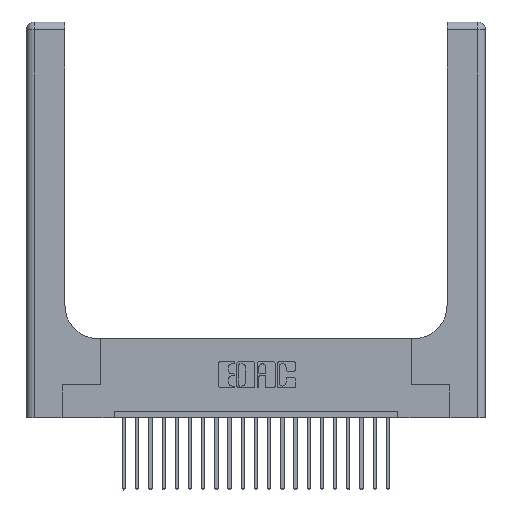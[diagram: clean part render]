
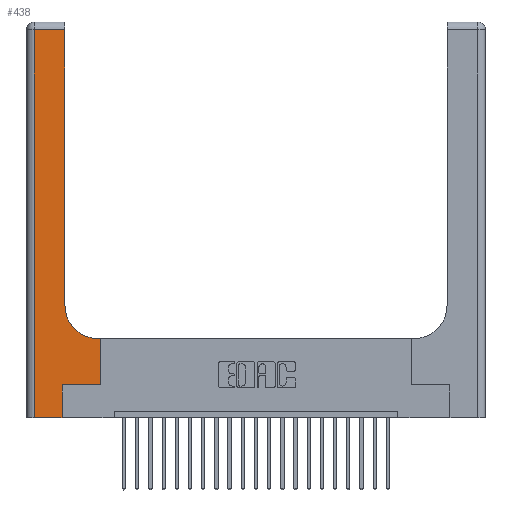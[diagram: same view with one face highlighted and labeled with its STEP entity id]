
A CAD part, top view. The second image highlights one B-rep face of the part: STEP entity #438.
In plain terms, the highlighted planar face has unit normal (0, 0, 1).
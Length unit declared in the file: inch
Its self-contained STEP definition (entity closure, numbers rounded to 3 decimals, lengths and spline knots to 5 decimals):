
#438 = ADVANCED_FACE ( 'NONE', ( #7470 ), #15779, .F. ) ;
#453 = VERTEX_POINT ( 'NONE', #10794 ) ;
#756 = EDGE_CURVE ( 'NONE', #19715, #3794, #6027, .T. ) ;
#1613 = DIRECTION ( 'NONE',  ( 0., -1., 0. ) ) ;
#1788 = EDGE_LOOP ( 'NONE', ( #12836, #7570, #6353, #3367, #19321, #16873, #14589, #3341, #20490 ) ) ;
#1799 = AXIS2_PLACEMENT_3D ( 'NONE', #7245, #14450, #12780 ) ;
#1943 = VERTEX_POINT ( 'NONE', #6002 ) ;
#2061 = CARTESIAN_POINT ( 'NONE',  ( 0.2915, 0.85, 0.37 ) ) ;
#3341 = ORIENTED_EDGE ( 'NONE', *, *, #756, .T. ) ;
#3367 = ORIENTED_EDGE ( 'NONE', *, *, #21802, .T. ) ;
#3630 = VERTEX_POINT ( 'NONE', #15208 ) ;
#3794 = VERTEX_POINT ( 'NONE', #13186 ) ;
#3799 = AXIS2_PLACEMENT_3D ( 'NONE', #9484, #14961, #5735 ) ;
#4421 = LINE ( 'NONE', #23392, #7592 ) ;
#4543 = LINE ( 'NONE', #18191, #22988 ) ;
#5642 = EDGE_CURVE ( 'NONE', #3794, #5722, #8721, .T. ) ;
#5643 = DIRECTION ( 'NONE',  ( -1., 0., 0. ) ) ;
#5722 = VERTEX_POINT ( 'NONE', #2061 ) ;
#5735 = DIRECTION ( 'NONE',  ( 1., 0., 0. ) ) ;
#5801 = CARTESIAN_POINT ( 'NONE',  ( 0.2915, 3., 0.37 ) ) ;
#5881 = CARTESIAN_POINT ( 'NONE',  ( 0.06, 0., 0.37 ) ) ;
#6002 = CARTESIAN_POINT ( 'NONE',  ( 0.269, 0.25, 0.37 ) ) ;
#6027 = LINE ( 'NONE', #17598, #14611 ) ;
#6353 = ORIENTED_EDGE ( 'NONE', *, *, #13974, .T. ) ;
#6705 = DIRECTION ( 'NONE',  ( 1., 0., 0. ) ) ;
#7245 = CARTESIAN_POINT ( 'NONE',  ( 0., 3., 0.37 ) ) ;
#7247 = CARTESIAN_POINT ( 'NONE',  ( 0.5585, 0.25, 0.37 ) ) ;
#7470 = FACE_OUTER_BOUND ( 'NONE', #1788, .T. ) ;
#7570 = ORIENTED_EDGE ( 'NONE', *, *, #15554, .T. ) ;
#7592 = VECTOR ( 'NONE', #21837, 39.37008 ) ;
#7974 = CARTESIAN_POINT ( 'NONE',  ( 0.269, 0., 0.37 ) ) ;
#8308 = VECTOR ( 'NONE', #5643, 39.37008 ) ;
#8721 = CIRCLE ( 'NONE', #3799, 0.25 ) ;
#8742 = VERTEX_POINT ( 'NONE', #5881 ) ;
#8880 = CARTESIAN_POINT ( 'NONE',  ( 0., 2.94, 0.37 ) ) ;
#8986 = VECTOR ( 'NONE', #1613, 39.37008 ) ;
#9078 = EDGE_CURVE ( 'NONE', #14714, #1943, #4543, .T. ) ;
#9465 = VECTOR ( 'NONE', #13879, 39.37008 ) ;
#9484 = CARTESIAN_POINT ( 'NONE',  ( 0.5415, 0.85, 0.37 ) ) ;
#9547 = DIRECTION ( 'NONE',  ( 0., 1., 0. ) ) ;
#10569 = CARTESIAN_POINT ( 'NONE',  ( 0.269, 0.25, 0.37 ) ) ;
#10794 = CARTESIAN_POINT ( 'NONE',  ( 0.2915, 2.94, 0.37 ) ) ;
#11045 = EDGE_CURVE ( 'NONE', #5722, #453, #16253, .T. ) ;
#11336 = CARTESIAN_POINT ( 'NONE',  ( 0.5585, 0.6, 0.37 ) ) ;
#11388 = VECTOR ( 'NONE', #9547, 39.37008 ) ;
#11629 = LINE ( 'NONE', #10569, #12191 ) ;
#11729 = EDGE_CURVE ( 'NONE', #14083, #19715, #4421, .T. ) ;
#12191 = VECTOR ( 'NONE', #6705, 39.37008 ) ;
#12325 = LINE ( 'NONE', #8880, #8308 ) ;
#12328 = DIRECTION ( 'NONE',  ( 0., 1., 0. ) ) ;
#12780 = DIRECTION ( 'NONE',  ( -1., 0., 0. ) ) ;
#12836 = ORIENTED_EDGE ( 'NONE', *, *, #11045, .T. ) ;
#13186 = CARTESIAN_POINT ( 'NONE',  ( 0.5415, 0.6, 0.37 ) ) ;
#13879 = DIRECTION ( 'NONE',  ( 1., 0., 0. ) ) ;
#13974 = EDGE_CURVE ( 'NONE', #3630, #8742, #19315, .T. ) ;
#14083 = VERTEX_POINT ( 'NONE', #7247 ) ;
#14313 = LINE ( 'NONE', #19346, #9465 ) ;
#14450 = DIRECTION ( 'NONE',  ( 0., 0., -1. ) ) ;
#14589 = ORIENTED_EDGE ( 'NONE', *, *, #11729, .T. ) ;
#14611 = VECTOR ( 'NONE', #23171, 39.37008 ) ;
#14714 = VERTEX_POINT ( 'NONE', #7974 ) ;
#14961 = DIRECTION ( 'NONE',  ( 0., 0., -1. ) ) ;
#15208 = CARTESIAN_POINT ( 'NONE',  ( 0.06, 2.94, 0.37 ) ) ;
#15554 = EDGE_CURVE ( 'NONE', #453, #3630, #12325, .T. ) ;
#15779 = PLANE ( 'NONE',  #1799 ) ;
#16253 = LINE ( 'NONE', #5801, #11388 ) ;
#16391 = CARTESIAN_POINT ( 'NONE',  ( 0.06, 3., 0.37 ) ) ;
#16873 = ORIENTED_EDGE ( 'NONE', *, *, #19189, .T. ) ;
#17598 = CARTESIAN_POINT ( 'NONE',  ( 0.2915, 0.6, 0.37 ) ) ;
#18191 = CARTESIAN_POINT ( 'NONE',  ( 0.269, 0., 0.37 ) ) ;
#19189 = EDGE_CURVE ( 'NONE', #1943, #14083, #11629, .T. ) ;
#19315 = LINE ( 'NONE', #16391, #8986 ) ;
#19321 = ORIENTED_EDGE ( 'NONE', *, *, #9078, .T. ) ;
#19346 = CARTESIAN_POINT ( 'NONE',  ( 0., 0., 0.37 ) ) ;
#19715 = VERTEX_POINT ( 'NONE', #11336 ) ;
#20490 = ORIENTED_EDGE ( 'NONE', *, *, #5642, .T. ) ;
#21802 = EDGE_CURVE ( 'NONE', #8742, #14714, #14313, .T. ) ;
#21837 = DIRECTION ( 'NONE',  ( 0., 1., 0. ) ) ;
#22988 = VECTOR ( 'NONE', #12328, 39.37008 ) ;
#23171 = DIRECTION ( 'NONE',  ( -1., 0., 0. ) ) ;
#23392 = CARTESIAN_POINT ( 'NONE',  ( 0.5585, 0.25, 0.37 ) ) ;
